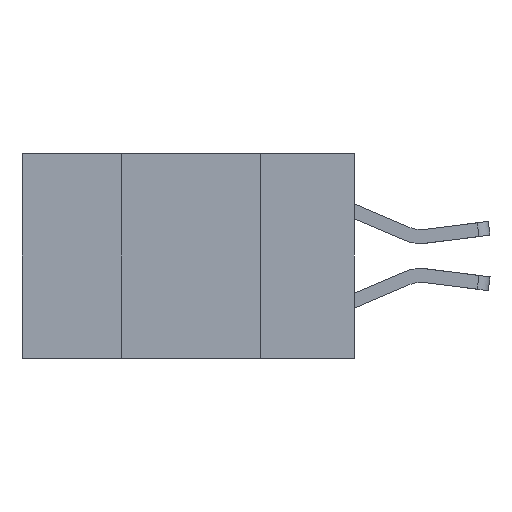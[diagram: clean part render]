
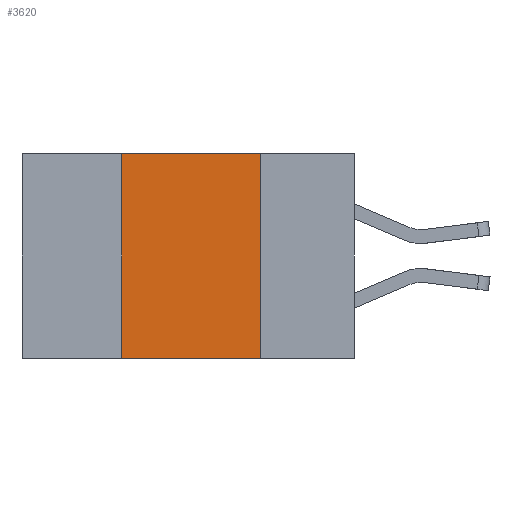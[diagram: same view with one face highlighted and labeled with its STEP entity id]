
A CAD part, left-side view. The second image highlights one B-rep face of the part: STEP entity #3620.
In plain terms, the highlighted planar face has unit normal (-1, 0, 0).
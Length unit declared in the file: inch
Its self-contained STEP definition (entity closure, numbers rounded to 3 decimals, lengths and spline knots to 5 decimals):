
#233 = EDGE_CURVE ( 'NONE', #2110, #8393, #8558, .T. ) ;
#346 = CARTESIAN_POINT ( 'NONE',  ( 0., 0.42, 0. ) ) ;
#438 = EDGE_CURVE ( 'NONE', #5159, #8393, #9135, .T. ) ;
#1346 = CARTESIAN_POINT ( 'NONE',  ( 0., 0.17, 0. ) ) ;
#1347 = VECTOR ( 'NONE', #7718, 39.37008 ) ;
#1693 = VERTEX_POINT ( 'NONE', #346 ) ;
#1697 = DIRECTION ( 'NONE',  ( 0., 0., -1. ) ) ;
#2110 = VERTEX_POINT ( 'NONE', #1346 ) ;
#2633 = ORIENTED_EDGE ( 'NONE', *, *, #438, .T. ) ;
#3573 = ORIENTED_EDGE ( 'NONE', *, *, #7419, .F. ) ;
#3620 = ADVANCED_FACE ( 'NONE', ( #8622 ), #8787, .F. ) ;
#3641 = ORIENTED_EDGE ( 'NONE', *, *, #233, .F. ) ;
#4248 = CARTESIAN_POINT ( 'NONE',  ( 0., 0.6, 0. ) ) ;
#4497 = EDGE_CURVE ( 'NONE', #5159, #1693, #7169, .T. ) ;
#5100 = VECTOR ( 'NONE', #8052, 39.37008 ) ;
#5159 = VERTEX_POINT ( 'NONE', #8813 ) ;
#5537 = ORIENTED_EDGE ( 'NONE', *, *, #4497, .F. ) ;
#5559 = EDGE_LOOP ( 'NONE', ( #3641, #3573, #5537, #2633 ) ) ;
#5888 = CARTESIAN_POINT ( 'NONE',  ( 0., 0.17, -0.37 ) ) ;
#6025 = CARTESIAN_POINT ( 'NONE',  ( 0., 0.17, -0.37 ) ) ;
#6300 = DIRECTION ( 'NONE',  ( 0., -1., 0. ) ) ;
#6632 = VECTOR ( 'NONE', #1697, 39.37008 ) ;
#6994 = CARTESIAN_POINT ( 'NONE',  ( 0., 0.6, 0. ) ) ;
#7169 = LINE ( 'NONE', #7730, #5100 ) ;
#7419 = EDGE_CURVE ( 'NONE', #1693, #2110, #7628, .T. ) ;
#7526 = CARTESIAN_POINT ( 'NONE',  ( 0., 0.6, -0.37 ) ) ;
#7540 = AXIS2_PLACEMENT_3D ( 'NONE', #4248, #8759, #9571 ) ;
#7628 = LINE ( 'NONE', #6994, #1347 ) ;
#7718 = DIRECTION ( 'NONE',  ( 0., -1., 0. ) ) ;
#7730 = CARTESIAN_POINT ( 'NONE',  ( 0., 0.42, -0.37 ) ) ;
#8052 = DIRECTION ( 'NONE',  ( 0., 0., 1. ) ) ;
#8393 = VERTEX_POINT ( 'NONE', #6025 ) ;
#8558 = LINE ( 'NONE', #5888, #6632 ) ;
#8622 = FACE_OUTER_BOUND ( 'NONE', #5559, .T. ) ;
#8759 = DIRECTION ( 'NONE',  ( 1., 0., 0. ) ) ;
#8787 = PLANE ( 'NONE',  #7540 ) ;
#8813 = CARTESIAN_POINT ( 'NONE',  ( 0., 0.42, -0.37 ) ) ;
#8903 = VECTOR ( 'NONE', #6300, 39.37008 ) ;
#9135 = LINE ( 'NONE', #7526, #8903 ) ;
#9571 = DIRECTION ( 'NONE',  ( 0., 0., -1. ) ) ;
